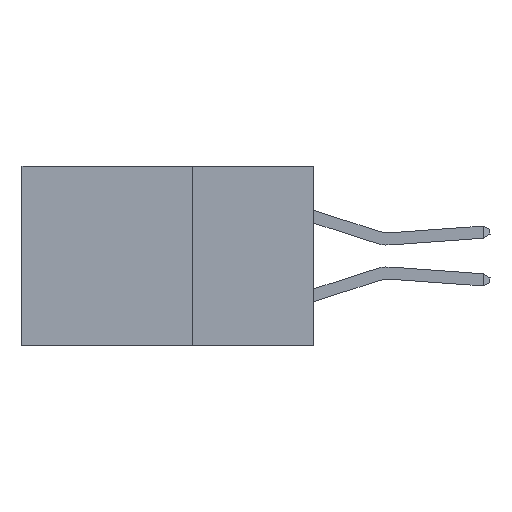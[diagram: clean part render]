
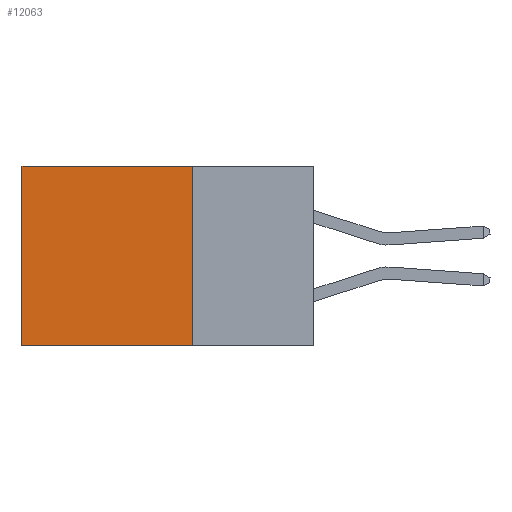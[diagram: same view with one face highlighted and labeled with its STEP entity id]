
A CAD part, left-side view. The second image highlights one B-rep face of the part: STEP entity #12063.
In plain terms, the highlighted planar face has unit normal (-1, 0, 0).
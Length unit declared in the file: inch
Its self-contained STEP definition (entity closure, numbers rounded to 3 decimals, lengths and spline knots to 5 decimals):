
#231 = CARTESIAN_POINT ( 'NONE',  ( 0.2875, 0.6, 0. ) ) ;
#529 = CARTESIAN_POINT ( 'NONE',  ( 0.2875, 0.6, 0. ) ) ;
#796 = CARTESIAN_POINT ( 'NONE',  ( 0.2875, 0.25, 0. ) ) ;
#1040 = CARTESIAN_POINT ( 'NONE',  ( 0.2875, 0.6, -0.37 ) ) ;
#1690 = VERTEX_POINT ( 'NONE', #2119 ) ;
#1884 = PLANE ( 'NONE',  #5443 ) ;
#2119 = CARTESIAN_POINT ( 'NONE',  ( 0.2875, 0.25, -0.37 ) ) ;
#2160 = VECTOR ( 'NONE', #10442, 39.37008 ) ;
#3705 = ORIENTED_EDGE ( 'NONE', *, *, #4598, .F. ) ;
#3862 = VECTOR ( 'NONE', #5683, 39.37008 ) ;
#3890 = ORIENTED_EDGE ( 'NONE', *, *, #4319, .F. ) ;
#4115 = EDGE_CURVE ( 'NONE', #10260, #12311, #5247, .T. ) ;
#4319 = EDGE_CURVE ( 'NONE', #1690, #12311, #12957, .T. ) ;
#4464 = CARTESIAN_POINT ( 'NONE',  ( 0.2875, 0.25, 0. ) ) ;
#4598 = EDGE_CURVE ( 'NONE', #9074, #1690, #6229, .T. ) ;
#4650 = CARTESIAN_POINT ( 'NONE',  ( 0.2875, 0.25, -0.37 ) ) ;
#4740 = EDGE_LOOP ( 'NONE', ( #6653, #3890, #3705, #11654 ) ) ;
#5061 = CARTESIAN_POINT ( 'NONE',  ( 0.2875, 0.25, 0. ) ) ;
#5247 = LINE ( 'NONE', #231, #3862 ) ;
#5443 = AXIS2_PLACEMENT_3D ( 'NONE', #13999, #12959, #7378 ) ;
#5683 = DIRECTION ( 'NONE',  ( 0., 0., -1. ) ) ;
#6229 = LINE ( 'NONE', #796, #6747 ) ;
#6653 = ORIENTED_EDGE ( 'NONE', *, *, #4115, .T. ) ;
#6747 = VECTOR ( 'NONE', #13977, 39.37008 ) ;
#6766 = VECTOR ( 'NONE', #12552, 39.37008 ) ;
#7378 = DIRECTION ( 'NONE',  ( 0., 0., -1. ) ) ;
#9074 = VERTEX_POINT ( 'NONE', #4464 ) ;
#9357 = EDGE_CURVE ( 'NONE', #9074, #10260, #10927, .T. ) ;
#10260 = VERTEX_POINT ( 'NONE', #529 ) ;
#10442 = DIRECTION ( 'NONE',  ( 0., 1., 0. ) ) ;
#10927 = LINE ( 'NONE', #5061, #2160 ) ;
#11615 = FACE_OUTER_BOUND ( 'NONE', #4740, .T. ) ;
#11654 = ORIENTED_EDGE ( 'NONE', *, *, #9357, .T. ) ;
#12063 = ADVANCED_FACE ( 'NONE', ( #11615 ), #1884, .F. ) ;
#12311 = VERTEX_POINT ( 'NONE', #1040 ) ;
#12552 = DIRECTION ( 'NONE',  ( 0., 1., 0. ) ) ;
#12957 = LINE ( 'NONE', #4650, #6766 ) ;
#12959 = DIRECTION ( 'NONE',  ( 1., 0., 0. ) ) ;
#13977 = DIRECTION ( 'NONE',  ( 0., 0., -1. ) ) ;
#13999 = CARTESIAN_POINT ( 'NONE',  ( 0.2875, 0.25, 0. ) ) ;
